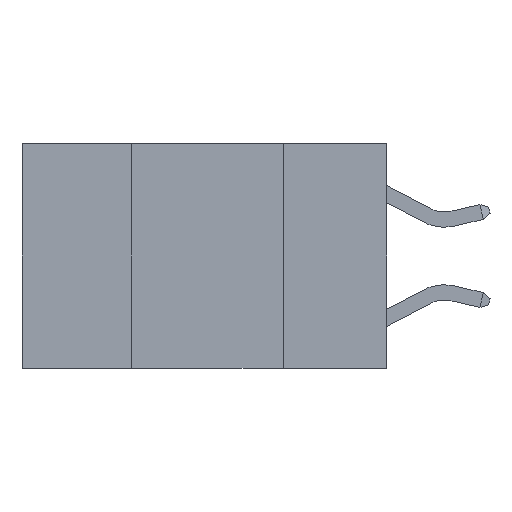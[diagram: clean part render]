
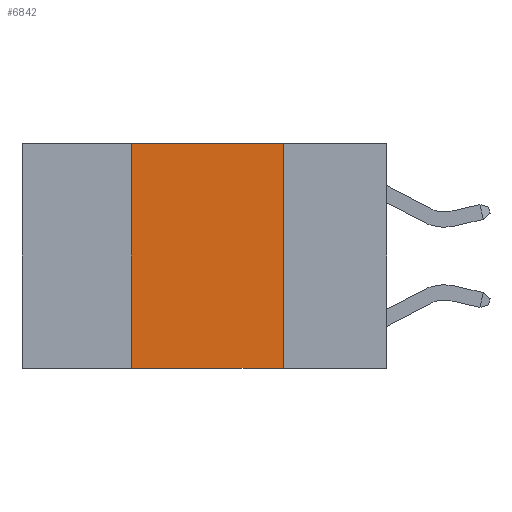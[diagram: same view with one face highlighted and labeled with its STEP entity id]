
A CAD part, left-side view. The second image highlights one B-rep face of the part: STEP entity #6842.
In plain terms, the highlighted planar face has unit normal (-1, 0, 0).
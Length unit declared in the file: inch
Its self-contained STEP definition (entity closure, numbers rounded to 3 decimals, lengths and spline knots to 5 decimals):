
#409 = PLANE ( 'NONE',  #11936 ) ;
#946 = ORIENTED_EDGE ( 'NONE', *, *, #6689, .F. ) ;
#1266 = CARTESIAN_POINT ( 'NONE',  ( 0., 0.6, 0. ) ) ;
#1356 = ORIENTED_EDGE ( 'NONE', *, *, #11436, .F. ) ;
#3035 = EDGE_LOOP ( 'NONE', ( #946, #7524, #1356, #12741 ) ) ;
#3712 = CARTESIAN_POINT ( 'NONE',  ( 0., 0.6, -0.37 ) ) ;
#3734 = VERTEX_POINT ( 'NONE', #4904 ) ;
#4105 = EDGE_CURVE ( 'NONE', #6547, #3734, #13570, .T. ) ;
#4542 = CARTESIAN_POINT ( 'NONE',  ( 0., 0.17, 0. ) ) ;
#4904 = CARTESIAN_POINT ( 'NONE',  ( 0., 0.17, -0.37 ) ) ;
#5486 = LINE ( 'NONE', #10756, #12381 ) ;
#6547 = VERTEX_POINT ( 'NONE', #8273 ) ;
#6559 = DIRECTION ( 'NONE',  ( 0., 0., -1. ) ) ;
#6689 = EDGE_CURVE ( 'NONE', #9994, #3734, #5486, .T. ) ;
#6842 = ADVANCED_FACE ( 'NONE', ( #10102 ), #409, .F. ) ;
#7085 = DIRECTION ( 'NONE',  ( 0., -1., 0. ) ) ;
#7524 = ORIENTED_EDGE ( 'NONE', *, *, #12454, .F. ) ;
#7634 = VECTOR ( 'NONE', #7085, 39.37008 ) ;
#7983 = DIRECTION ( 'NONE',  ( 0., 0., -1. ) ) ;
#8184 = DIRECTION ( 'NONE',  ( 0., 0., 1. ) ) ;
#8273 = CARTESIAN_POINT ( 'NONE',  ( 0., 0.42, -0.37 ) ) ;
#9994 = VERTEX_POINT ( 'NONE', #4542 ) ;
#10102 = FACE_OUTER_BOUND ( 'NONE', #3035, .T. ) ;
#10625 = LINE ( 'NONE', #12515, #11787 ) ;
#10756 = CARTESIAN_POINT ( 'NONE',  ( 0., 0.17, 0. ) ) ;
#10882 = VERTEX_POINT ( 'NONE', #11123 ) ;
#11123 = CARTESIAN_POINT ( 'NONE',  ( 0., 0.42, 0. ) ) ;
#11292 = LINE ( 'NONE', #12478, #13337 ) ;
#11436 = EDGE_CURVE ( 'NONE', #6547, #10882, #11292, .T. ) ;
#11787 = VECTOR ( 'NONE', #12579, 39.37008 ) ;
#11936 = AXIS2_PLACEMENT_3D ( 'NONE', #1266, #12142, #7983 ) ;
#12142 = DIRECTION ( 'NONE',  ( 1., 0., 0. ) ) ;
#12381 = VECTOR ( 'NONE', #6559, 39.37008 ) ;
#12454 = EDGE_CURVE ( 'NONE', #10882, #9994, #10625, .T. ) ;
#12478 = CARTESIAN_POINT ( 'NONE',  ( 0., 0.42, 0. ) ) ;
#12515 = CARTESIAN_POINT ( 'NONE',  ( 0., 0.6, 0. ) ) ;
#12579 = DIRECTION ( 'NONE',  ( 0., -1., 0. ) ) ;
#12741 = ORIENTED_EDGE ( 'NONE', *, *, #4105, .T. ) ;
#13337 = VECTOR ( 'NONE', #8184, 39.37008 ) ;
#13570 = LINE ( 'NONE', #3712, #7634 ) ;
